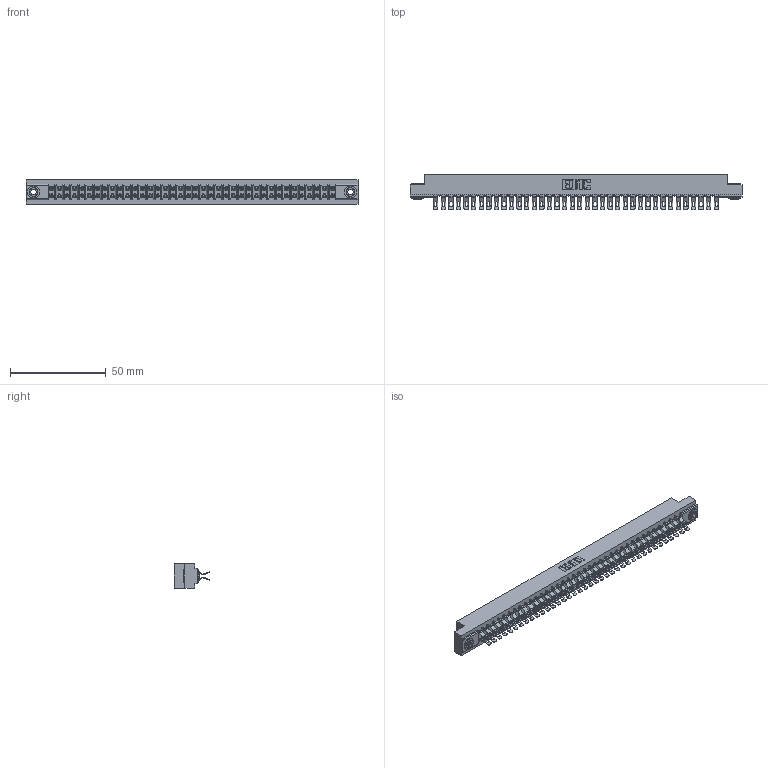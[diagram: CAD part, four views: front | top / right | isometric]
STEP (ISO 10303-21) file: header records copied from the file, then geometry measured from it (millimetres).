
FILE_DESCRIPTION (( 'STEP AP203' ), '1' );
FILE_NAME ('307-076-555-203.STEP', '2019-09-06T22:08:44', ( '' ), ( '' ), 'SwSTEP 2.0', 'SolidWorks 2016', '' );
FILE_SCHEMA (( 'CONFIG_CONTROL_DESIGN' ));
Length unit declared in the file: inch
Products named in the file (4): 307-290-001_555; 307 Part_.156 Dia Mounting Holes; 307-076-555-203; 345-250-002_345-250-002-102
Assembly tree (79 placements, depth 2):
  307-076-555-203
    307 Part_.156 Dia Mounting Holes
    307-290-001_555  x76
    345-250-002_345-250-002-102  x2
Bounding box: 173.58 x 18.75 x 12.7 mm (x, y, z)
Volume: 18658 mm3; surface area: 24255.6 mm2
Topology: 79 solids, 79 shells, 4845 faces, 14191 edges, 9250 vertices
Faces by surface type: plane 2678, cylinder 2081, sphere 78, cone 8
Entity records: 35888 total; most frequent: CARTESIAN_POINT 5859, ORIENTED_EDGE 5800, DIRECTION 5762, EDGE_CURVE 2900, VECTOR 2204, LINE 2204, VERTEX_POINT 1876, AXIS2_PLACEMENT_3D 1779
